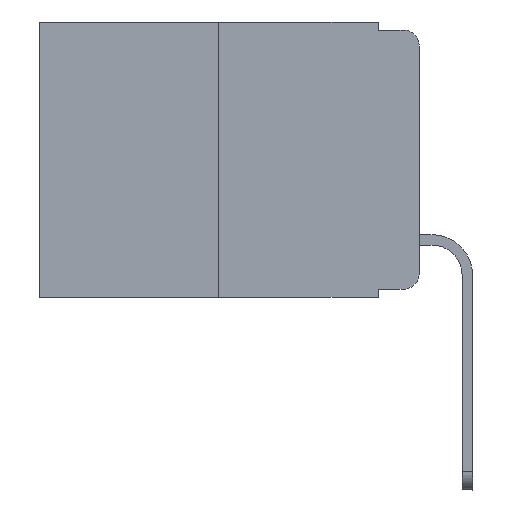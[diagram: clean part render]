
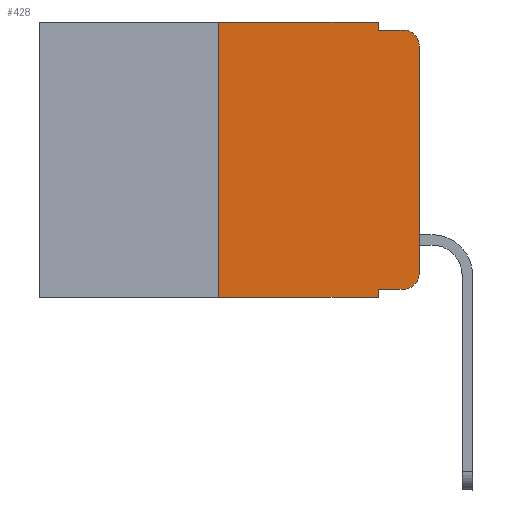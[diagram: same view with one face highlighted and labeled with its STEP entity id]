
A CAD part, left-side view. The second image highlights one B-rep face of the part: STEP entity #428.
In plain terms, the highlighted planar face has unit normal (-1, 0, 0).
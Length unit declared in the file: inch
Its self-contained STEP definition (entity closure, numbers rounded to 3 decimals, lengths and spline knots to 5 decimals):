
#163 = CIRCLE ( 'NONE', #9044, 0.02 ) ;
#309 = FACE_OUTER_BOUND ( 'NONE', #9084, .T. ) ;
#428 = ADVANCED_FACE ( 'NONE', ( #309 ), #1348, .F. ) ;
#484 = AXIS2_PLACEMENT_3D ( 'NONE', #6290, #5089, #9154 ) ;
#536 = CARTESIAN_POINT ( 'NONE',  ( 0., 0.051, -0.01 ) ) ;
#552 = CARTESIAN_POINT ( 'NONE',  ( 0., 0.02, -0.333 ) ) ;
#674 = DIRECTION ( 'NONE',  ( 0., 0., 1. ) ) ;
#825 = VECTOR ( 'NONE', #4509, 39.37008 ) ;
#889 = EDGE_CURVE ( 'NONE', #8365, #4990, #11501, .T. ) ;
#954 = VECTOR ( 'NONE', #3890, 39.37008 ) ;
#1348 = PLANE ( 'NONE',  #12876 ) ;
#1356 = CARTESIAN_POINT ( 'NONE',  ( 0., 0.051, 0. ) ) ;
#1482 = CARTESIAN_POINT ( 'NONE',  ( 0., 0.473, 0. ) ) ;
#1619 = ORIENTED_EDGE ( 'NONE', *, *, #7179, .F. ) ;
#1757 = ORIENTED_EDGE ( 'NONE', *, *, #11032, .F. ) ;
#1947 = CARTESIAN_POINT ( 'NONE',  ( 0., 0.051, -0.01 ) ) ;
#2073 = VECTOR ( 'NONE', #2457, 39.37008 ) ;
#2303 = DIRECTION ( 'NONE',  ( 0., 0., -1. ) ) ;
#2457 = DIRECTION ( 'NONE',  ( 0., 0., -1. ) ) ;
#2627 = VERTEX_POINT ( 'NONE', #8193 ) ;
#2662 = DIRECTION ( 'NONE',  ( 0., 0., -1. ) ) ;
#3238 = ORIENTED_EDGE ( 'NONE', *, *, #9893, .T. ) ;
#3318 = VERTEX_POINT ( 'NONE', #7569 ) ;
#3549 = CARTESIAN_POINT ( 'NONE',  ( 0., 0.473, -0.343 ) ) ;
#3672 = LINE ( 'NONE', #3549, #7745 ) ;
#3778 = VECTOR ( 'NONE', #8172, 39.37008 ) ;
#3890 = DIRECTION ( 'NONE',  ( 0., 0., 1. ) ) ;
#4017 = VERTEX_POINT ( 'NONE', #7410 ) ;
#4090 = VERTEX_POINT ( 'NONE', #536 ) ;
#4509 = DIRECTION ( 'NONE',  ( 0., -1., 0. ) ) ;
#4626 = LINE ( 'NONE', #8679, #6086 ) ;
#4737 = CARTESIAN_POINT ( 'NONE',  ( 0., 0.02, -0.01 ) ) ;
#4980 = CARTESIAN_POINT ( 'NONE',  ( 0., 0., -0.313 ) ) ;
#4990 = VERTEX_POINT ( 'NONE', #552 ) ;
#4997 = ORIENTED_EDGE ( 'NONE', *, *, #9877, .F. ) ;
#5025 = CARTESIAN_POINT ( 'NONE',  ( 0., 0.051, -0.333 ) ) ;
#5089 = DIRECTION ( 'NONE',  ( -1., 0., 0. ) ) ;
#5281 = EDGE_CURVE ( 'NONE', #4017, #12026, #5545, .T. ) ;
#5435 = DIRECTION ( 'NONE',  ( 0., -1., 0. ) ) ;
#5545 = CIRCLE ( 'NONE', #484, 0.02 ) ;
#6046 = ORIENTED_EDGE ( 'NONE', *, *, #5281, .T. ) ;
#6086 = VECTOR ( 'NONE', #674, 39.37008 ) ;
#6290 = CARTESIAN_POINT ( 'NONE',  ( 0., 0.02, -0.03 ) ) ;
#6512 = DIRECTION ( 'NONE',  ( -1., 0., 0. ) ) ;
#6649 = DIRECTION ( 'NONE',  ( 0., 0., -1. ) ) ;
#6661 = DIRECTION ( 'NONE',  ( 0., -1., 0. ) ) ;
#6699 = LINE ( 'NONE', #8473, #2073 ) ;
#7037 = ORIENTED_EDGE ( 'NONE', *, *, #889, .T. ) ;
#7179 = EDGE_CURVE ( 'NONE', #3318, #2627, #12131, .T. ) ;
#7410 = CARTESIAN_POINT ( 'NONE',  ( 0., 0., -0.03 ) ) ;
#7569 = CARTESIAN_POINT ( 'NONE',  ( 0., 0.25, -0.343 ) ) ;
#7745 = VECTOR ( 'NONE', #6661, 39.37008 ) ;
#7866 = VERTEX_POINT ( 'NONE', #10696 ) ;
#8107 = LINE ( 'NONE', #1947, #3778 ) ;
#8172 = DIRECTION ( 'NONE',  ( 0., -1., 0. ) ) ;
#8193 = CARTESIAN_POINT ( 'NONE',  ( 0., 0.25, 0. ) ) ;
#8365 = VERTEX_POINT ( 'NONE', #5025 ) ;
#8425 = LINE ( 'NONE', #1482, #825 ) ;
#8473 = CARTESIAN_POINT ( 'NONE',  ( 0., 0.051, 0. ) ) ;
#8679 = CARTESIAN_POINT ( 'NONE',  ( 0., 0., 0. ) ) ;
#8987 = VERTEX_POINT ( 'NONE', #10759 ) ;
#9044 = AXIS2_PLACEMENT_3D ( 'NONE', #12628, #6512, #2662 ) ;
#9050 = EDGE_CURVE ( 'NONE', #3318, #7866, #3672, .T. ) ;
#9084 = EDGE_LOOP ( 'NONE', ( #3238, #6046, #12680, #1757, #10655, #1619, #11050, #4997, #7037, #10915 ) ) ;
#9154 = DIRECTION ( 'NONE',  ( 0., 0., -1. ) ) ;
#9188 = VERTEX_POINT ( 'NONE', #4980 ) ;
#9432 = EDGE_CURVE ( 'NONE', #4990, #9188, #163, .T. ) ;
#9750 = VECTOR ( 'NONE', #5435, 39.37008 ) ;
#9877 = EDGE_CURVE ( 'NONE', #8365, #7866, #6699, .T. ) ;
#9893 = EDGE_CURVE ( 'NONE', #9188, #4017, #4626, .T. ) ;
#10188 = CARTESIAN_POINT ( 'NONE',  ( 0., 0.25, 0. ) ) ;
#10655 = ORIENTED_EDGE ( 'NONE', *, *, #12748, .F. ) ;
#10696 = CARTESIAN_POINT ( 'NONE',  ( 0., 0.051, -0.343 ) ) ;
#10753 = VECTOR ( 'NONE', #2303, 39.37008 ) ;
#10759 = CARTESIAN_POINT ( 'NONE',  ( 0., 0.051, 0. ) ) ;
#10915 = ORIENTED_EDGE ( 'NONE', *, *, #9432, .T. ) ;
#11032 = EDGE_CURVE ( 'NONE', #8987, #4090, #11345, .T. ) ;
#11050 = ORIENTED_EDGE ( 'NONE', *, *, #9050, .T. ) ;
#11345 = LINE ( 'NONE', #1356, #10753 ) ;
#11501 = LINE ( 'NONE', #12681, #9750 ) ;
#11772 = DIRECTION ( 'NONE',  ( 1., 0., 0. ) ) ;
#12026 = VERTEX_POINT ( 'NONE', #4737 ) ;
#12131 = LINE ( 'NONE', #10188, #954 ) ;
#12370 = CARTESIAN_POINT ( 'NONE',  ( 0., 0.473, 0. ) ) ;
#12565 = EDGE_CURVE ( 'NONE', #4090, #12026, #8107, .T. ) ;
#12628 = CARTESIAN_POINT ( 'NONE',  ( 0., 0.02, -0.313 ) ) ;
#12680 = ORIENTED_EDGE ( 'NONE', *, *, #12565, .F. ) ;
#12681 = CARTESIAN_POINT ( 'NONE',  ( 0., 0.051, -0.333 ) ) ;
#12748 = EDGE_CURVE ( 'NONE', #2627, #8987, #8425, .T. ) ;
#12876 = AXIS2_PLACEMENT_3D ( 'NONE', #12370, #11772, #6649 ) ;
